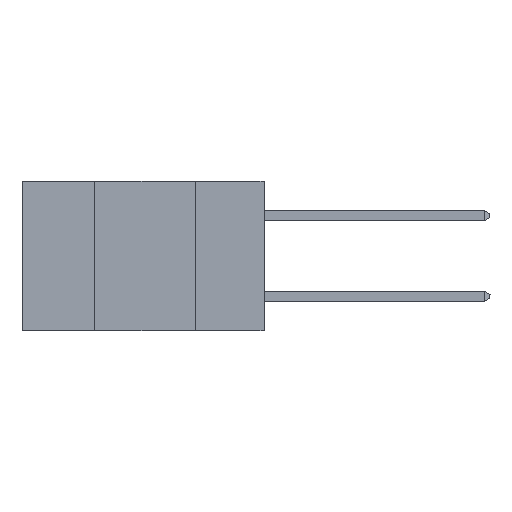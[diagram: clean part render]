
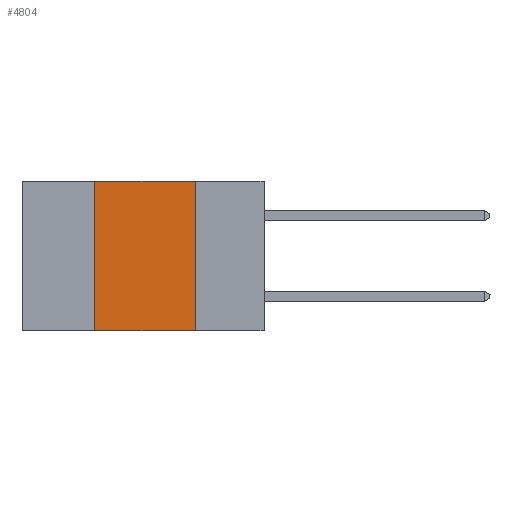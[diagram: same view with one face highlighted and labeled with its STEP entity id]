
A CAD part, left-side view. The second image highlights one B-rep face of the part: STEP entity #4804.
In plain terms, the highlighted planar face has unit normal (-1, 0, 0).
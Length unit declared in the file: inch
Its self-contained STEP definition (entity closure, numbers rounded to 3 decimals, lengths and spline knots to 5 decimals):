
#96 = CARTESIAN_POINT ( 'NONE',  ( 0., 0.42, 0. ) ) ;
#976 = ORIENTED_EDGE ( 'NONE', *, *, #6306, .F. ) ;
#1450 = VERTEX_POINT ( 'NONE', #15338 ) ;
#1706 = CARTESIAN_POINT ( 'NONE',  ( 0., 0.17, 0. ) ) ;
#2300 = VECTOR ( 'NONE', #15123, 39.37008 ) ;
#3277 = CARTESIAN_POINT ( 'NONE',  ( 0., 0.6, 0. ) ) ;
#3369 = EDGE_CURVE ( 'NONE', #1450, #11740, #12612, .T. ) ;
#3499 = CARTESIAN_POINT ( 'NONE',  ( 0., 0.6, -0.37 ) ) ;
#4736 = EDGE_CURVE ( 'NONE', #11740, #9041, #16226, .T. ) ;
#4804 = ADVANCED_FACE ( 'NONE', ( #13211 ), #13360, .F. ) ;
#5067 = CARTESIAN_POINT ( 'NONE',  ( 0., 0.17, -0.37 ) ) ;
#6306 = EDGE_CURVE ( 'NONE', #8043, #1450, #8562, .T. ) ;
#7625 = DIRECTION ( 'NONE',  ( 0., 0., 1. ) ) ;
#8043 = VERTEX_POINT ( 'NONE', #16185 ) ;
#8325 = CARTESIAN_POINT ( 'NONE',  ( 0., 0.17, 0. ) ) ;
#8562 = LINE ( 'NONE', #96, #9365 ) ;
#8919 = AXIS2_PLACEMENT_3D ( 'NONE', #3277, #12340, #9709 ) ;
#9041 = VERTEX_POINT ( 'NONE', #5067 ) ;
#9280 = ORIENTED_EDGE ( 'NONE', *, *, #14191, .T. ) ;
#9365 = VECTOR ( 'NONE', #7625, 39.37008 ) ;
#9709 = DIRECTION ( 'NONE',  ( 0., 0., -1. ) ) ;
#10233 = ORIENTED_EDGE ( 'NONE', *, *, #3369, .F. ) ;
#11420 = CARTESIAN_POINT ( 'NONE',  ( 0., 0.6, 0. ) ) ;
#11740 = VERTEX_POINT ( 'NONE', #8325 ) ;
#12010 = VECTOR ( 'NONE', #12068, 39.37008 ) ;
#12068 = DIRECTION ( 'NONE',  ( 0., 0., -1. ) ) ;
#12340 = DIRECTION ( 'NONE',  ( 1., 0., 0. ) ) ;
#12612 = LINE ( 'NONE', #11420, #2300 ) ;
#12958 = ORIENTED_EDGE ( 'NONE', *, *, #4736, .F. ) ;
#13194 = LINE ( 'NONE', #3499, #14201 ) ;
#13211 = FACE_OUTER_BOUND ( 'NONE', #14220, .T. ) ;
#13360 = PLANE ( 'NONE',  #8919 ) ;
#14191 = EDGE_CURVE ( 'NONE', #8043, #9041, #13194, .T. ) ;
#14201 = VECTOR ( 'NONE', #16233, 39.37008 ) ;
#14220 = EDGE_LOOP ( 'NONE', ( #12958, #10233, #976, #9280 ) ) ;
#15123 = DIRECTION ( 'NONE',  ( 0., -1., 0. ) ) ;
#15338 = CARTESIAN_POINT ( 'NONE',  ( 0., 0.42, 0. ) ) ;
#16185 = CARTESIAN_POINT ( 'NONE',  ( 0., 0.42, -0.37 ) ) ;
#16226 = LINE ( 'NONE', #1706, #12010 ) ;
#16233 = DIRECTION ( 'NONE',  ( 0., -1., 0. ) ) ;
